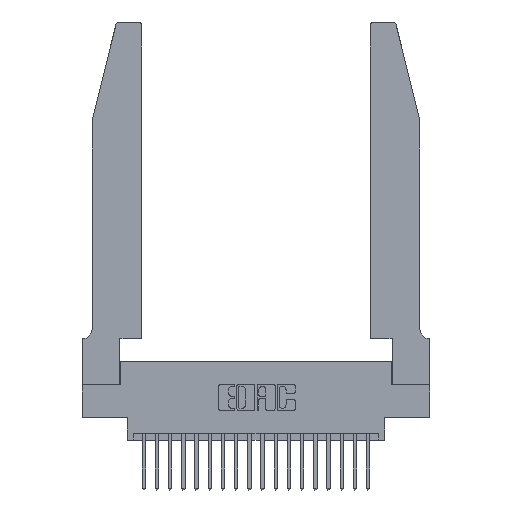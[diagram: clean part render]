
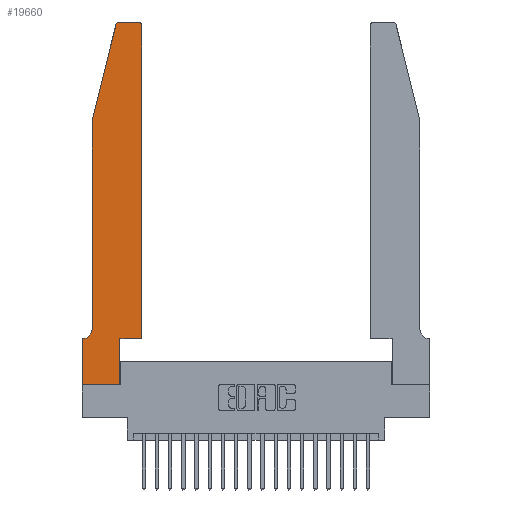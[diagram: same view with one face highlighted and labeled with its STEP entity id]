
A CAD part, top view. The second image highlights one B-rep face of the part: STEP entity #19660.
In plain terms, the highlighted planar face has unit normal (0, 0, 1).
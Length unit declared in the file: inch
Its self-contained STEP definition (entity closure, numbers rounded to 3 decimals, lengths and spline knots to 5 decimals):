
#166 = EDGE_CURVE ( 'NONE', #3516, #2885, #1775, .T. ) ;
#174 = LINE ( 'NONE', #9862, #16874 ) ;
#507 = EDGE_CURVE ( 'NONE', #4065, #1521, #6895, .T. ) ;
#859 = CARTESIAN_POINT ( 'NONE',  ( 0.2865, 0., 0.37 ) ) ;
#1369 = ORIENTED_EDGE ( 'NONE', *, *, #18394, .T. ) ;
#1508 = VECTOR ( 'NONE', #19228, 39.37008 ) ;
#1521 = VERTEX_POINT ( 'NONE', #19491 ) ;
#1743 = CARTESIAN_POINT ( 'NONE',  ( 0.0055, 0.35, 0.37 ) ) ;
#1775 = CIRCLE ( 'NONE', #8998, 0.03 ) ;
#1780 = DIRECTION ( 'NONE',  ( 1., 0., 0. ) ) ;
#1855 = ORIENTED_EDGE ( 'NONE', *, *, #16855, .T. ) ;
#1925 = DIRECTION ( 'NONE',  ( 0., 0., 1. ) ) ;
#1940 = CARTESIAN_POINT ( 'NONE',  ( 0.2865, 0.35, 0.37 ) ) ;
#2226 = ORIENTED_EDGE ( 'NONE', *, *, #11880, .T. ) ;
#2480 = CARTESIAN_POINT ( 'NONE',  ( 0.2865, 0.35, 0.37 ) ) ;
#2571 = LINE ( 'NONE', #19005, #1508 ) ;
#2720 = ORIENTED_EDGE ( 'NONE', *, *, #166, .T. ) ;
#2885 = VERTEX_POINT ( 'NONE', #11572 ) ;
#3174 = FACE_OUTER_BOUND ( 'NONE', #20889, .T. ) ;
#3354 = DIRECTION ( 'NONE',  ( -1., 0., 0. ) ) ;
#3358 = EDGE_CURVE ( 'NONE', #9727, #4065, #16148, .T. ) ;
#3366 = EDGE_CURVE ( 'NONE', #20828, #14318, #7028, .T. ) ;
#3448 = AXIS2_PLACEMENT_3D ( 'NONE', #9580, #6279, #9662 ) ;
#3516 = VERTEX_POINT ( 'NONE', #9881 ) ;
#3643 = VERTEX_POINT ( 'NONE', #12035 ) ;
#3696 = CARTESIAN_POINT ( 'NONE',  ( 0.4505, 0.35, 0.37 ) ) ;
#3732 = DIRECTION ( 'NONE',  ( 1., 0., 0. ) ) ;
#3833 = ORIENTED_EDGE ( 'NONE', *, *, #3366, .T. ) ;
#4065 = VERTEX_POINT ( 'NONE', #19783 ) ;
#4360 = DIRECTION ( 'NONE',  ( -0.239, -0.971, 0. ) ) ;
#4470 = DIRECTION ( 'NONE',  ( 1., 0., 0. ) ) ;
#5816 = VECTOR ( 'NONE', #11780, 39.37008 ) ;
#6065 = VECTOR ( 'NONE', #3732, 39.37008 ) ;
#6165 = DIRECTION ( 'NONE',  ( 0., 0., -1. ) ) ;
#6229 = VECTOR ( 'NONE', #4360, 39.37008 ) ;
#6233 = CARTESIAN_POINT ( 'NONE',  ( 0.284, 2.72, 0.37 ) ) ;
#6279 = DIRECTION ( 'NONE',  ( 0., 0., 1. ) ) ;
#6326 = VERTEX_POINT ( 'NONE', #14005 ) ;
#6589 = EDGE_CURVE ( 'NONE', #11167, #6326, #2571, .T. ) ;
#6617 = CARTESIAN_POINT ( 'NONE',  ( 0.0755, 2., 0.37 ) ) ;
#6844 = DIRECTION ( 'NONE',  ( -1., 0., 0. ) ) ;
#6895 = LINE ( 'NONE', #6617, #5816 ) ;
#7028 = LINE ( 'NONE', #2480, #7552 ) ;
#7231 = ORIENTED_EDGE ( 'NONE', *, *, #3358, .T. ) ;
#7552 = VECTOR ( 'NONE', #21329, 39.37008 ) ;
#7818 = LINE ( 'NONE', #12152, #10767 ) ;
#8124 = ORIENTED_EDGE ( 'NONE', *, *, #19083, .T. ) ;
#8225 = LINE ( 'NONE', #14064, #6065 ) ;
#8269 = CARTESIAN_POINT ( 'NONE',  ( 0.2605, 2.75, 0.37 ) ) ;
#8781 = ORIENTED_EDGE ( 'NONE', *, *, #6589, .T. ) ;
#8880 = DIRECTION ( 'NONE',  ( 0., 1., 0. ) ) ;
#8998 = AXIS2_PLACEMENT_3D ( 'NONE', #10300, #1925, #1780 ) ;
#9088 = LINE ( 'NONE', #8269, #19534 ) ;
#9580 = CARTESIAN_POINT ( 'NONE',  ( 0., 0.35, 0.37 ) ) ;
#9662 = DIRECTION ( 'NONE',  ( 1., 0., 0. ) ) ;
#9727 = VERTEX_POINT ( 'NONE', #17113 ) ;
#9862 = CARTESIAN_POINT ( 'NONE',  ( 0., 0., 0.37 ) ) ;
#9881 = CARTESIAN_POINT ( 'NONE',  ( 0.4505, 2.72, 0.37 ) ) ;
#10300 = CARTESIAN_POINT ( 'NONE',  ( 0.4205, 2.72, 0.37 ) ) ;
#10418 = EDGE_CURVE ( 'NONE', #1521, #15293, #15359, .T. ) ;
#10767 = VECTOR ( 'NONE', #8880, 39.37008 ) ;
#11167 = VERTEX_POINT ( 'NONE', #11767 ) ;
#11358 = DIRECTION ( 'NONE',  ( 1., 0., 0. ) ) ;
#11572 = CARTESIAN_POINT ( 'NONE',  ( 0.4205, 2.75, 0.37 ) ) ;
#11767 = CARTESIAN_POINT ( 'NONE',  ( 0., 0.35, 0.37 ) ) ;
#11780 = DIRECTION ( 'NONE',  ( 0., -1., 0. ) ) ;
#11880 = EDGE_CURVE ( 'NONE', #15293, #11167, #20639, .T. ) ;
#12035 = CARTESIAN_POINT ( 'NONE',  ( 0.284, 2.75, 0.37 ) ) ;
#12152 = CARTESIAN_POINT ( 'NONE',  ( 0.4505, 0.35, 0.37 ) ) ;
#13139 = VECTOR ( 'NONE', #3354, 39.37008 ) ;
#14005 = CARTESIAN_POINT ( 'NONE',  ( 0., 0., 0.37 ) ) ;
#14064 = CARTESIAN_POINT ( 'NONE',  ( 0.4505, 0.35, 0.37 ) ) ;
#14318 = VERTEX_POINT ( 'NONE', #1940 ) ;
#14672 = CARTESIAN_POINT ( 'NONE',  ( 0.0755, 2., 0.37 ) ) ;
#15293 = VERTEX_POINT ( 'NONE', #1743 ) ;
#15359 = CIRCLE ( 'NONE', #18165, 0.07 ) ;
#16133 = CIRCLE ( 'NONE', #17545, 0.03 ) ;
#16148 = LINE ( 'NONE', #14672, #6229 ) ;
#16440 = CARTESIAN_POINT ( 'NONE',  ( 0.0055, 0.42, 0.37 ) ) ;
#16516 = DIRECTION ( 'NONE',  ( 0., 0., 1. ) ) ;
#16855 = EDGE_CURVE ( 'NONE', #17505, #3516, #7818, .T. ) ;
#16874 = VECTOR ( 'NONE', #11358, 39.37008 ) ;
#17113 = CARTESIAN_POINT ( 'NONE',  ( 0.25487, 2.72718, 0.37 ) ) ;
#17505 = VERTEX_POINT ( 'NONE', #3696 ) ;
#17545 = AXIS2_PLACEMENT_3D ( 'NONE', #6233, #16516, #4470 ) ;
#17657 = ORIENTED_EDGE ( 'NONE', *, *, #507, .T. ) ;
#18134 = DIRECTION ( 'NONE',  ( -1., 0., 0. ) ) ;
#18165 = AXIS2_PLACEMENT_3D ( 'NONE', #16440, #6165, #18134 ) ;
#18328 = PLANE ( 'NONE',  #3448 ) ;
#18394 = EDGE_CURVE ( 'NONE', #6326, #20828, #174, .T. ) ;
#18673 = ORIENTED_EDGE ( 'NONE', *, *, #20523, .T. ) ;
#19005 = CARTESIAN_POINT ( 'NONE',  ( 0., 0., 0.37 ) ) ;
#19083 = EDGE_CURVE ( 'NONE', #3643, #9727, #16133, .T. ) ;
#19228 = DIRECTION ( 'NONE',  ( 0., -1., 0. ) ) ;
#19491 = CARTESIAN_POINT ( 'NONE',  ( 0.0755, 0.42, 0.37 ) ) ;
#19534 = VECTOR ( 'NONE', #6844, 39.37008 ) ;
#19660 = ADVANCED_FACE ( 'NONE', ( #3174 ), #18328, .T. ) ;
#19783 = CARTESIAN_POINT ( 'NONE',  ( 0.0755, 2., 0.37 ) ) ;
#19804 = ORIENTED_EDGE ( 'NONE', *, *, #10418, .T. ) ;
#20523 = EDGE_CURVE ( 'NONE', #2885, #3643, #9088, .T. ) ;
#20611 = ORIENTED_EDGE ( 'NONE', *, *, #21649, .T. ) ;
#20639 = LINE ( 'NONE', #22219, #13139 ) ;
#20828 = VERTEX_POINT ( 'NONE', #859 ) ;
#20889 = EDGE_LOOP ( 'NONE', ( #18673, #8124, #7231, #17657, #19804, #2226, #8781, #1369, #3833, #20611, #1855, #2720 ) ) ;
#21329 = DIRECTION ( 'NONE',  ( 0., 1., 0. ) ) ;
#21649 = EDGE_CURVE ( 'NONE', #14318, #17505, #8225, .T. ) ;
#22219 = CARTESIAN_POINT ( 'NONE',  ( 0.0755, 0.35, 0.37 ) ) ;
